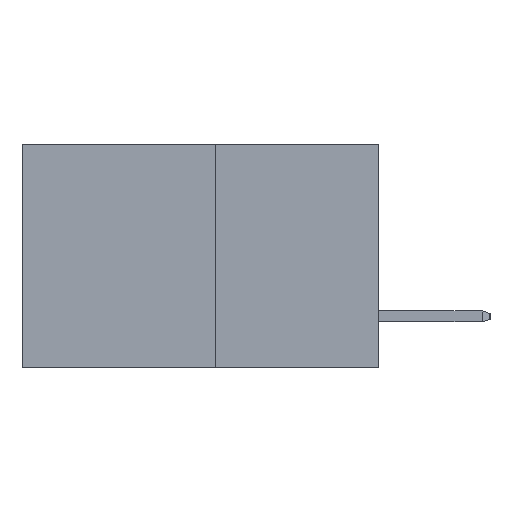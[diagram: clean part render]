
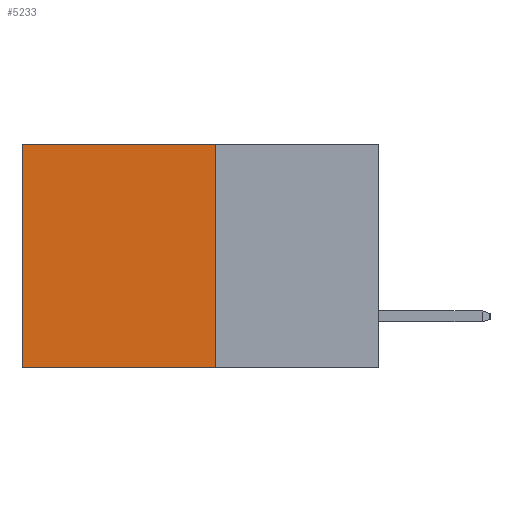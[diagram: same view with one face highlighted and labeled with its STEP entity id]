
A CAD part, left-side view. The second image highlights one B-rep face of the part: STEP entity #5233.
In plain terms, the highlighted planar face has unit normal (-1, 0, 0).
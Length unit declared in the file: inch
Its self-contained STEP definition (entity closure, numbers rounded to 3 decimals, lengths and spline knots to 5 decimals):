
#113 = LINE ( 'NONE', #8800, #11520 ) ;
#908 = FACE_OUTER_BOUND ( 'NONE', #2940, .T. ) ;
#1843 = LINE ( 'NONE', #7367, #7922 ) ;
#1962 = ORIENTED_EDGE ( 'NONE', *, *, #12200, .F. ) ;
#2205 = DIRECTION ( 'NONE',  ( 0., 0., -1. ) ) ;
#2604 = LINE ( 'NONE', #12368, #14098 ) ;
#2940 = EDGE_LOOP ( 'NONE', ( #10651, #3786, #1962, #13868 ) ) ;
#3028 = VERTEX_POINT ( 'NONE', #12490 ) ;
#3786 = ORIENTED_EDGE ( 'NONE', *, *, #3999, .F. ) ;
#3844 = PLANE ( 'NONE',  #9436 ) ;
#3881 = CARTESIAN_POINT ( 'NONE',  ( 0.277, 0.27, -0.37 ) ) ;
#3999 = EDGE_CURVE ( 'NONE', #13374, #7504, #2604, .T. ) ;
#4521 = EDGE_CURVE ( 'NONE', #6915, #3028, #1843, .T. ) ;
#5233 = ADVANCED_FACE ( 'NONE', ( #908 ), #3844, .F. ) ;
#5679 = CARTESIAN_POINT ( 'NONE',  ( 0.277, 0.27, -0.37 ) ) ;
#5902 = DIRECTION ( 'NONE',  ( 0., 0., -1. ) ) ;
#5905 = DIRECTION ( 'NONE',  ( 1., 0., 0. ) ) ;
#6875 = EDGE_CURVE ( 'NONE', #3028, #7504, #113, .T. ) ;
#6915 = VERTEX_POINT ( 'NONE', #8492 ) ;
#7221 = DIRECTION ( 'NONE',  ( 0., 1., 0. ) ) ;
#7367 = CARTESIAN_POINT ( 'NONE',  ( 0.277, 0.27, 0. ) ) ;
#7504 = VERTEX_POINT ( 'NONE', #13720 ) ;
#7882 = CARTESIAN_POINT ( 'NONE',  ( 0.277, 0.27, -0.37 ) ) ;
#7922 = VECTOR ( 'NONE', #7221, 39.37008 ) ;
#8492 = CARTESIAN_POINT ( 'NONE',  ( 0.277, 0.27, 0. ) ) ;
#8682 = DIRECTION ( 'NONE',  ( 0., 1., 0. ) ) ;
#8746 = DIRECTION ( 'NONE',  ( 0., 0., -1. ) ) ;
#8800 = CARTESIAN_POINT ( 'NONE',  ( 0.277, 0.59, -0.37 ) ) ;
#9179 = VECTOR ( 'NONE', #2205, 39.37008 ) ;
#9436 = AXIS2_PLACEMENT_3D ( 'NONE', #3881, #5905, #5902 ) ;
#9558 = LINE ( 'NONE', #7882, #9179 ) ;
#10651 = ORIENTED_EDGE ( 'NONE', *, *, #6875, .T. ) ;
#11520 = VECTOR ( 'NONE', #8746, 39.37008 ) ;
#12200 = EDGE_CURVE ( 'NONE', #6915, #13374, #9558, .T. ) ;
#12368 = CARTESIAN_POINT ( 'NONE',  ( 0.277, 0.27, -0.37 ) ) ;
#12490 = CARTESIAN_POINT ( 'NONE',  ( 0.277, 0.59, 0. ) ) ;
#13374 = VERTEX_POINT ( 'NONE', #5679 ) ;
#13720 = CARTESIAN_POINT ( 'NONE',  ( 0.277, 0.59, -0.37 ) ) ;
#13868 = ORIENTED_EDGE ( 'NONE', *, *, #4521, .T. ) ;
#14098 = VECTOR ( 'NONE', #8682, 39.37008 ) ;
